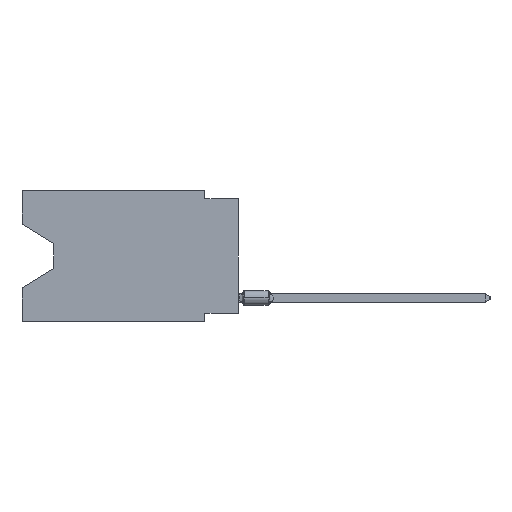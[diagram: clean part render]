
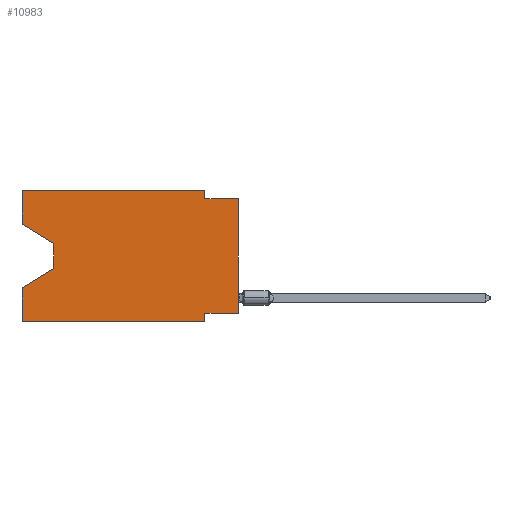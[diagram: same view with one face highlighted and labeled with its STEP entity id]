
A CAD part, left-side view. The second image highlights one B-rep face of the part: STEP entity #10983.
In plain terms, the highlighted planar face has unit normal (-1, 0, 0).
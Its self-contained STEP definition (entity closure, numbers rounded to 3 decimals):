
#132 = LINE ( 'NONE', #34798, #24210 ) ;
#368 = CARTESIAN_POINT ( 'NONE',  ( 0., 16.383, 0. ) ) ;
#412 = VERTEX_POINT ( 'NONE', #7658 ) ;
#679 = CARTESIAN_POINT ( 'NONE',  ( 0., 0., -0.635 ) ) ;
#980 = DIRECTION ( 'NONE',  ( 0., -1., 0. ) ) ;
#1578 = VECTOR ( 'NONE', #1856, 1000. ) ;
#1615 = VERTEX_POINT ( 'NONE', #6548 ) ;
#1755 = VECTOR ( 'NONE', #19086, 1000. ) ;
#1856 = DIRECTION ( 'NONE',  ( 0., 0., -1. ) ) ;
#2041 = CARTESIAN_POINT ( 'NONE',  ( 0., 2.54, -9.906 ) ) ;
#2623 = CARTESIAN_POINT ( 'NONE',  ( 0., 2.54, -9.271 ) ) ;
#3634 = CARTESIAN_POINT ( 'NONE',  ( 0., 16.383, 0. ) ) ;
#4190 = VECTOR ( 'NONE', #15491, 1000. ) ;
#5044 = DIRECTION ( 'NONE',  ( 0., -1., 0. ) ) ;
#6088 = LINE ( 'NONE', #20848, #10294 ) ;
#6399 = VERTEX_POINT ( 'NONE', #8590 ) ;
#6548 = CARTESIAN_POINT ( 'NONE',  ( 0., 2.54, -0.635 ) ) ;
#7077 = ORIENTED_EDGE ( 'NONE', *, *, #18438, .F. ) ;
#7358 = ORIENTED_EDGE ( 'NONE', *, *, #7395, .F. ) ;
#7395 = EDGE_CURVE ( 'NONE', #1615, #31882, #26940, .T. ) ;
#7529 = CARTESIAN_POINT ( 'NONE',  ( 0., 16.383, -2.546 ) ) ;
#7658 = CARTESIAN_POINT ( 'NONE',  ( 0., 13.97, -5.893 ) ) ;
#7780 = LINE ( 'NONE', #19340, #30428 ) ;
#8237 = LINE ( 'NONE', #36327, #16891 ) ;
#8273 = ORIENTED_EDGE ( 'NONE', *, *, #13899, .T. ) ;
#8590 = CARTESIAN_POINT ( 'NONE',  ( 0., 16.383, -7.36 ) ) ;
#8678 = DIRECTION ( 'NONE',  ( 0., -1., 0. ) ) ;
#8800 = DIRECTION ( 'NONE',  ( 0., 0., -1. ) ) ;
#9245 = VERTEX_POINT ( 'NONE', #19175 ) ;
#9250 = CARTESIAN_POINT ( 'NONE',  ( 0., 13.97, -5.893 ) ) ;
#9436 = LINE ( 'NONE', #368, #18162 ) ;
#9566 = CARTESIAN_POINT ( 'NONE',  ( 0., 16.383, -9.906 ) ) ;
#10294 = VECTOR ( 'NONE', #12145, 1000. ) ;
#10324 = VECTOR ( 'NONE', #23082, 1000. ) ;
#10455 = LINE ( 'NONE', #24856, #34074 ) ;
#10934 = LINE ( 'NONE', #2041, #1578 ) ;
#10983 = ADVANCED_FACE ( 'NONE', ( #16959 ), #37440, .F. ) ;
#11836 = CARTESIAN_POINT ( 'NONE',  ( 0., 16.383, 0. ) ) ;
#12018 = ORIENTED_EDGE ( 'NONE', *, *, #30792, .F. ) ;
#12028 = ORIENTED_EDGE ( 'NONE', *, *, #16378, .T. ) ;
#12145 = DIRECTION ( 'NONE',  ( 0., 0., 1. ) ) ;
#12792 = CARTESIAN_POINT ( 'NONE',  ( 0., 16.383, -2.546 ) ) ;
#13728 = EDGE_CURVE ( 'NONE', #26065, #412, #10455, .T. ) ;
#13899 = EDGE_CURVE ( 'NONE', #15118, #31882, #7780, .T. ) ;
#14159 = VERTEX_POINT ( 'NONE', #3634 ) ;
#14488 = ORIENTED_EDGE ( 'NONE', *, *, #20014, .F. ) ;
#15118 = VERTEX_POINT ( 'NONE', #19145 ) ;
#15491 = DIRECTION ( 'NONE',  ( 0., 0.855, -0.519 ) ) ;
#15985 = EDGE_CURVE ( 'NONE', #412, #6399, #35235, .T. ) ;
#16378 = EDGE_CURVE ( 'NONE', #24159, #33602, #8237, .T. ) ;
#16891 = VECTOR ( 'NONE', #5044, 1000. ) ;
#16959 = FACE_OUTER_BOUND ( 'NONE', #22206, .T. ) ;
#17265 = EDGE_CURVE ( 'NONE', #14159, #9245, #9436, .T. ) ;
#17857 = LINE ( 'NONE', #7529, #1755 ) ;
#17956 = CARTESIAN_POINT ( 'NONE',  ( 0., 16.383, 0. ) ) ;
#18162 = VECTOR ( 'NONE', #8678, 1000. ) ;
#18438 = EDGE_CURVE ( 'NONE', #26580, #14159, #6088, .T. ) ;
#19086 = DIRECTION ( 'NONE',  ( 0., -0.855, -0.519 ) ) ;
#19145 = CARTESIAN_POINT ( 'NONE',  ( 0., 0., -9.271 ) ) ;
#19175 = CARTESIAN_POINT ( 'NONE',  ( 0., 2.54, 0. ) ) ;
#19340 = CARTESIAN_POINT ( 'NONE',  ( 0., 0., 0. ) ) ;
#19828 = LINE ( 'NONE', #37475, #30592 ) ;
#19893 = AXIS2_PLACEMENT_3D ( 'NONE', #11836, #31573, #28915 ) ;
#20014 = EDGE_CURVE ( 'NONE', #9245, #1615, #132, .T. ) ;
#20553 = EDGE_CURVE ( 'NONE', #24159, #6399, #31812, .T. ) ;
#20755 = ORIENTED_EDGE ( 'NONE', *, *, #17265, .F. ) ;
#20848 = CARTESIAN_POINT ( 'NONE',  ( 0., 16.383, 0. ) ) ;
#21403 = CARTESIAN_POINT ( 'NONE',  ( 0., 0., -0.635 ) ) ;
#22206 = EDGE_LOOP ( 'NONE', ( #22552, #28289, #35338, #26577, #12028, #12018, #35781, #8273, #7358, #14488, #20755, #7077 ) ) ;
#22552 = ORIENTED_EDGE ( 'NONE', *, *, #25825, .T. ) ;
#23082 = DIRECTION ( 'NONE',  ( 0., 0., 1. ) ) ;
#23458 = CARTESIAN_POINT ( 'NONE',  ( 0., 2.54, -9.906 ) ) ;
#23729 = VECTOR ( 'NONE', #980, 1000. ) ;
#24159 = VERTEX_POINT ( 'NONE', #9566 ) ;
#24210 = VECTOR ( 'NONE', #8800, 1000. ) ;
#24856 = CARTESIAN_POINT ( 'NONE',  ( 0., 13.97, -4.013 ) ) ;
#25825 = EDGE_CURVE ( 'NONE', #26580, #26065, #17857, .T. ) ;
#26065 = VERTEX_POINT ( 'NONE', #32567 ) ;
#26577 = ORIENTED_EDGE ( 'NONE', *, *, #20553, .F. ) ;
#26580 = VERTEX_POINT ( 'NONE', #12792 ) ;
#26940 = LINE ( 'NONE', #21403, #23729 ) ;
#28264 = DIRECTION ( 'NONE',  ( 0., 0., 1. ) ) ;
#28289 = ORIENTED_EDGE ( 'NONE', *, *, #13728, .T. ) ;
#28580 = DIRECTION ( 'NONE',  ( 0., 1., 0. ) ) ;
#28915 = DIRECTION ( 'NONE',  ( 0., 0., -1. ) ) ;
#30428 = VECTOR ( 'NONE', #28264, 1000. ) ;
#30592 = VECTOR ( 'NONE', #28580, 1000. ) ;
#30792 = EDGE_CURVE ( 'NONE', #30891, #33602, #10934, .T. ) ;
#30891 = VERTEX_POINT ( 'NONE', #2623 ) ;
#31183 = EDGE_CURVE ( 'NONE', #15118, #30891, #19828, .T. ) ;
#31573 = DIRECTION ( 'NONE',  ( 1., 0., 0. ) ) ;
#31812 = LINE ( 'NONE', #17956, #10324 ) ;
#31882 = VERTEX_POINT ( 'NONE', #679 ) ;
#32567 = CARTESIAN_POINT ( 'NONE',  ( 0., 13.97, -4.013 ) ) ;
#33602 = VERTEX_POINT ( 'NONE', #23458 ) ;
#34074 = VECTOR ( 'NONE', #36989, 1000. ) ;
#34798 = CARTESIAN_POINT ( 'NONE',  ( 0., 2.54, 0. ) ) ;
#35235 = LINE ( 'NONE', #9250, #4190 ) ;
#35338 = ORIENTED_EDGE ( 'NONE', *, *, #15985, .T. ) ;
#35781 = ORIENTED_EDGE ( 'NONE', *, *, #31183, .F. ) ;
#36327 = CARTESIAN_POINT ( 'NONE',  ( 0., 16.383, -9.906 ) ) ;
#36989 = DIRECTION ( 'NONE',  ( 0., 0., -1. ) ) ;
#37440 = PLANE ( 'NONE',  #19893 ) ;
#37475 = CARTESIAN_POINT ( 'NONE',  ( 0., 0., -9.271 ) ) ;
